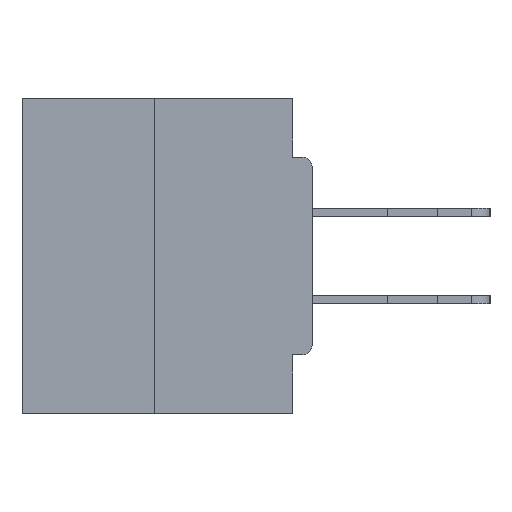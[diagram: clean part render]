
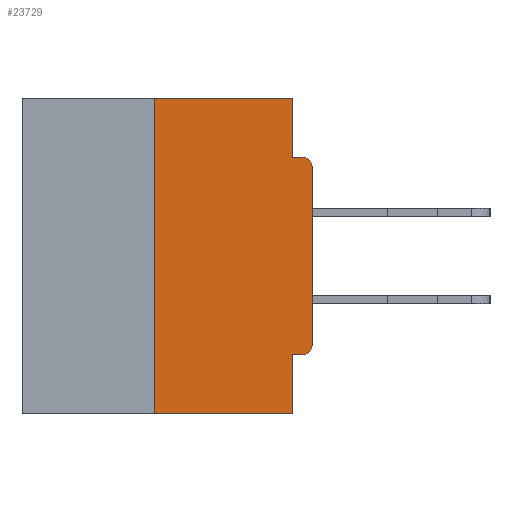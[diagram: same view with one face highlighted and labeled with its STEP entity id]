
A CAD part, left-side view. The second image highlights one B-rep face of the part: STEP entity #23729.
In plain terms, the highlighted planar face has unit normal (-1, 0, 0).
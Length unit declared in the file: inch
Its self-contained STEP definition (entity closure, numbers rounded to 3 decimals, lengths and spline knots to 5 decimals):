
#132 = CARTESIAN_POINT ( 'NONE',  ( 0., 0.031, 0. ) ) ;
#540 = VECTOR ( 'NONE', #21345, 39.37008 ) ;
#737 = CARTESIAN_POINT ( 'NONE',  ( 0., 0., -0.4065 ) ) ;
#901 = CARTESIAN_POINT ( 'NONE',  ( 0., 0., -0.3915 ) ) ;
#941 = CARTESIAN_POINT ( 'NONE',  ( 0., 0.031, -0.5 ) ) ;
#1417 = EDGE_CURVE ( 'NONE', #4339, #31774, #25029, .T. ) ;
#1900 = VECTOR ( 'NONE', #7462, 39.37008 ) ;
#2253 = VERTEX_POINT ( 'NONE', #12862 ) ;
#2553 = DIRECTION ( 'NONE',  ( 0., 0., -1. ) ) ;
#2809 = AXIS2_PLACEMENT_3D ( 'NONE', #26020, #18177, #2553 ) ;
#4125 = DIRECTION ( 'NONE',  ( 1., 0., 0. ) ) ;
#4151 = FACE_OUTER_BOUND ( 'NONE', #11095, .T. ) ;
#4183 = VECTOR ( 'NONE', #7260, 39.37008 ) ;
#4339 = VERTEX_POINT ( 'NONE', #31864 ) ;
#5245 = ORIENTED_EDGE ( 'NONE', *, *, #32493, .F. ) ;
#5480 = EDGE_CURVE ( 'NONE', #6125, #33576, #24700, .T. ) ;
#6125 = VERTEX_POINT ( 'NONE', #13223 ) ;
#7034 = VECTOR ( 'NONE', #20231, 39.37008 ) ;
#7235 = LINE ( 'NONE', #737, #22754 ) ;
#7260 = DIRECTION ( 'NONE',  ( 0., 0., -1. ) ) ;
#7462 = DIRECTION ( 'NONE',  ( 0., -1., 0. ) ) ;
#7510 = CARTESIAN_POINT ( 'NONE',  ( 0., 0.25, 0. ) ) ;
#7882 = ORIENTED_EDGE ( 'NONE', *, *, #1417, .T. ) ;
#7980 = CARTESIAN_POINT ( 'NONE',  ( 0., 0.015, -0.1085 ) ) ;
#8948 = CIRCLE ( 'NONE', #26824, 0.015 ) ;
#9139 = CARTESIAN_POINT ( 'NONE',  ( 0., 0.031, -0.4065 ) ) ;
#9158 = CARTESIAN_POINT ( 'NONE',  ( 0., 0., -0.1085 ) ) ;
#9520 = LINE ( 'NONE', #15778, #4183 ) ;
#10744 = VECTOR ( 'NONE', #30104, 39.37008 ) ;
#11095 = EDGE_LOOP ( 'NONE', ( #14667, #22819, #23695, #5245, #27185, #7882, #31133, #24860, #27171, #26961 ) ) ;
#12004 = DIRECTION ( 'NONE',  ( 0., 0., -1. ) ) ;
#12377 = VECTOR ( 'NONE', #29987, 39.37008 ) ;
#12862 = CARTESIAN_POINT ( 'NONE',  ( 0., 0.015, -0.0935 ) ) ;
#13223 = CARTESIAN_POINT ( 'NONE',  ( 0., 0.25, -0.5 ) ) ;
#14283 = LINE ( 'NONE', #30364, #20866 ) ;
#14667 = ORIENTED_EDGE ( 'NONE', *, *, #29339, .F. ) ;
#15199 = CARTESIAN_POINT ( 'NONE',  ( 0., 0.46, 0. ) ) ;
#15648 = CARTESIAN_POINT ( 'NONE',  ( 0., 0.25, 0. ) ) ;
#15778 = CARTESIAN_POINT ( 'NONE',  ( 0., 0.031, 0. ) ) ;
#15823 = DIRECTION ( 'NONE',  ( 0., 0., -1. ) ) ;
#15993 = VERTEX_POINT ( 'NONE', #132 ) ;
#16245 = CARTESIAN_POINT ( 'NONE',  ( 0., 0.031, -0.0935 ) ) ;
#16387 = LINE ( 'NONE', #33570, #7034 ) ;
#16743 = DIRECTION ( 'NONE',  ( 0., 1., 0. ) ) ;
#17756 = AXIS2_PLACEMENT_3D ( 'NONE', #22635, #4125, #12004 ) ;
#18177 = DIRECTION ( 'NONE',  ( -1., 0., 0. ) ) ;
#19317 = EDGE_CURVE ( 'NONE', #33531, #2253, #14283, .T. ) ;
#19719 = EDGE_CURVE ( 'NONE', #21909, #2253, #8948, .T. ) ;
#20231 = DIRECTION ( 'NONE',  ( 0., 0., 1. ) ) ;
#20531 = LINE ( 'NONE', #24911, #12377 ) ;
#20866 = VECTOR ( 'NONE', #30246, 39.37008 ) ;
#21007 = EDGE_CURVE ( 'NONE', #4339, #25022, #7235, .T. ) ;
#21079 = LINE ( 'NONE', #15199, #1900 ) ;
#21345 = DIRECTION ( 'NONE',  ( 0., 0., 1. ) ) ;
#21909 = VERTEX_POINT ( 'NONE', #9158 ) ;
#22635 = CARTESIAN_POINT ( 'NONE',  ( 0., 0.46, 0. ) ) ;
#22754 = VECTOR ( 'NONE', #16743, 39.37008 ) ;
#22819 = ORIENTED_EDGE ( 'NONE', *, *, #31674, .F. ) ;
#23313 = EDGE_CURVE ( 'NONE', #15993, #33531, #9520, .T. ) ;
#23695 = ORIENTED_EDGE ( 'NONE', *, *, #5480, .T. ) ;
#23729 = ADVANCED_FACE ( 'NONE', ( #4151 ), #30265, .F. ) ;
#23800 = EDGE_CURVE ( 'NONE', #31774, #21909, #16387, .T. ) ;
#24700 = LINE ( 'NONE', #27459, #10744 ) ;
#24747 = LINE ( 'NONE', #15648, #540 ) ;
#24860 = ORIENTED_EDGE ( 'NONE', *, *, #19719, .T. ) ;
#24911 = CARTESIAN_POINT ( 'NONE',  ( 0., 0.031, -0.5 ) ) ;
#25022 = VERTEX_POINT ( 'NONE', #9139 ) ;
#25029 = CIRCLE ( 'NONE', #2809, 0.015 ) ;
#26020 = CARTESIAN_POINT ( 'NONE',  ( 0., 0.015, -0.3915 ) ) ;
#26824 = AXIS2_PLACEMENT_3D ( 'NONE', #7980, #31600, #15823 ) ;
#26961 = ORIENTED_EDGE ( 'NONE', *, *, #23313, .F. ) ;
#27171 = ORIENTED_EDGE ( 'NONE', *, *, #19317, .F. ) ;
#27185 = ORIENTED_EDGE ( 'NONE', *, *, #21007, .F. ) ;
#27459 = CARTESIAN_POINT ( 'NONE',  ( 0., 0.46, -0.5 ) ) ;
#29339 = EDGE_CURVE ( 'NONE', #30817, #15993, #21079, .T. ) ;
#29987 = DIRECTION ( 'NONE',  ( 0., 0., -1. ) ) ;
#30104 = DIRECTION ( 'NONE',  ( 0., -1., 0. ) ) ;
#30246 = DIRECTION ( 'NONE',  ( 0., -1., 0. ) ) ;
#30265 = PLANE ( 'NONE',  #17756 ) ;
#30364 = CARTESIAN_POINT ( 'NONE',  ( 0., 0., -0.0935 ) ) ;
#30817 = VERTEX_POINT ( 'NONE', #7510 ) ;
#31133 = ORIENTED_EDGE ( 'NONE', *, *, #23800, .T. ) ;
#31600 = DIRECTION ( 'NONE',  ( -1., 0., 0. ) ) ;
#31674 = EDGE_CURVE ( 'NONE', #6125, #30817, #24747, .T. ) ;
#31774 = VERTEX_POINT ( 'NONE', #901 ) ;
#31864 = CARTESIAN_POINT ( 'NONE',  ( 0., 0.015, -0.4065 ) ) ;
#32493 = EDGE_CURVE ( 'NONE', #25022, #33576, #20531, .T. ) ;
#33531 = VERTEX_POINT ( 'NONE', #16245 ) ;
#33570 = CARTESIAN_POINT ( 'NONE',  ( 0., 0., 0. ) ) ;
#33576 = VERTEX_POINT ( 'NONE', #941 ) ;
